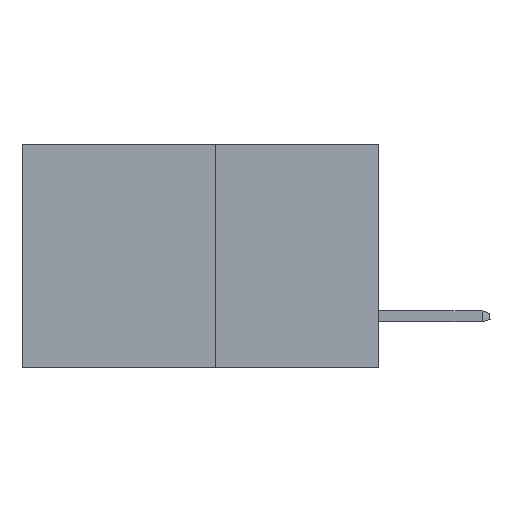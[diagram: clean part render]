
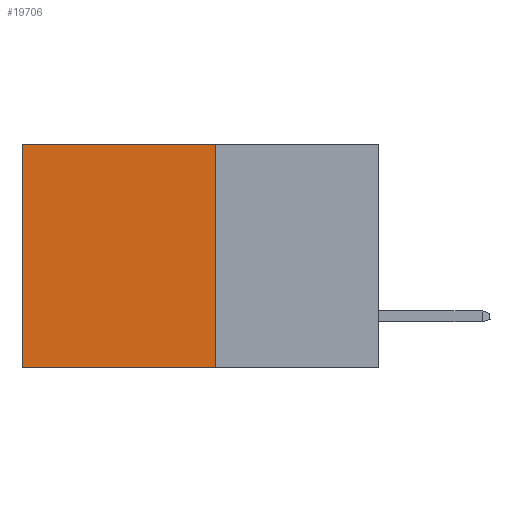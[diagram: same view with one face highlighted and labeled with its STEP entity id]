
A CAD part, left-side view. The second image highlights one B-rep face of the part: STEP entity #19706.
In plain terms, the highlighted planar face has unit normal (-1, 0, 0).
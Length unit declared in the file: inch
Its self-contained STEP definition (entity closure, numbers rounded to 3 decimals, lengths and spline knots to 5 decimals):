
#145 = LINE ( 'NONE', #16660, #19540 ) ;
#828 = PLANE ( 'NONE',  #4241 ) ;
#1101 = LINE ( 'NONE', #17036, #9999 ) ;
#1870 = DIRECTION ( 'NONE',  ( 0., 0., -1. ) ) ;
#2460 = ORIENTED_EDGE ( 'NONE', *, *, #6138, .T. ) ;
#2912 = VECTOR ( 'NONE', #1870, 39.37008 ) ;
#4188 = VERTEX_POINT ( 'NONE', #18629 ) ;
#4241 = AXIS2_PLACEMENT_3D ( 'NONE', #10337, #23306, #12251 ) ;
#6129 = EDGE_CURVE ( 'NONE', #4188, #10827, #145, .T. ) ;
#6138 = EDGE_CURVE ( 'NONE', #7767, #6635, #10808, .T. ) ;
#6635 = VERTEX_POINT ( 'NONE', #10656 ) ;
#7127 = FACE_OUTER_BOUND ( 'NONE', #22836, .T. ) ;
#7767 = VERTEX_POINT ( 'NONE', #22269 ) ;
#8970 = CARTESIAN_POINT ( 'NONE',  ( 0.277, 0.59, -0.37 ) ) ;
#9565 = ORIENTED_EDGE ( 'NONE', *, *, #21876, .F. ) ;
#9999 = VECTOR ( 'NONE', #15239, 39.37008 ) ;
#10337 = CARTESIAN_POINT ( 'NONE',  ( 0.277, 0.27, -0.37 ) ) ;
#10656 = CARTESIAN_POINT ( 'NONE',  ( 0.277, 0.59, 0. ) ) ;
#10808 = LINE ( 'NONE', #16114, #14624 ) ;
#10827 = VERTEX_POINT ( 'NONE', #8970 ) ;
#11609 = ORIENTED_EDGE ( 'NONE', *, *, #15923, .T. ) ;
#12251 = DIRECTION ( 'NONE',  ( 0., 0., -1. ) ) ;
#12796 = ORIENTED_EDGE ( 'NONE', *, *, #6129, .F. ) ;
#12912 = LINE ( 'NONE', #24179, #2912 ) ;
#14624 = VECTOR ( 'NONE', #16086, 39.37008 ) ;
#15239 = DIRECTION ( 'NONE',  ( 0., 0., -1. ) ) ;
#15923 = EDGE_CURVE ( 'NONE', #6635, #10827, #1101, .T. ) ;
#16086 = DIRECTION ( 'NONE',  ( 0., 1., 0. ) ) ;
#16114 = CARTESIAN_POINT ( 'NONE',  ( 0.277, 0.27, 0. ) ) ;
#16299 = DIRECTION ( 'NONE',  ( 0., 1., 0. ) ) ;
#16660 = CARTESIAN_POINT ( 'NONE',  ( 0.277, 0.27, -0.37 ) ) ;
#17036 = CARTESIAN_POINT ( 'NONE',  ( 0.277, 0.59, -0.37 ) ) ;
#18629 = CARTESIAN_POINT ( 'NONE',  ( 0.277, 0.27, -0.37 ) ) ;
#19540 = VECTOR ( 'NONE', #16299, 39.37008 ) ;
#19706 = ADVANCED_FACE ( 'NONE', ( #7127 ), #828, .F. ) ;
#21876 = EDGE_CURVE ( 'NONE', #7767, #4188, #12912, .T. ) ;
#22269 = CARTESIAN_POINT ( 'NONE',  ( 0.277, 0.27, 0. ) ) ;
#22836 = EDGE_LOOP ( 'NONE', ( #11609, #12796, #9565, #2460 ) ) ;
#23306 = DIRECTION ( 'NONE',  ( 1., 0., 0. ) ) ;
#24179 = CARTESIAN_POINT ( 'NONE',  ( 0.277, 0.27, -0.37 ) ) ;
